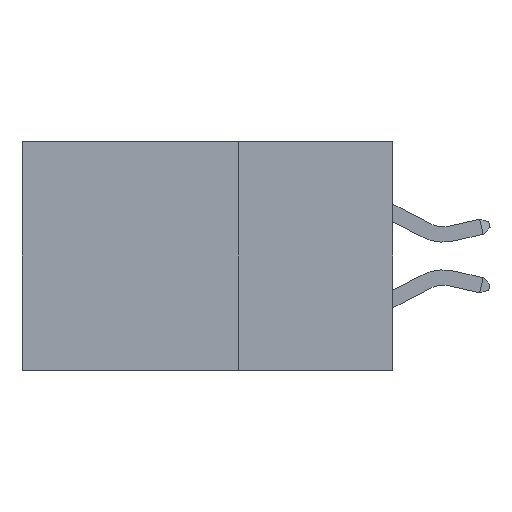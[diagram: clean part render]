
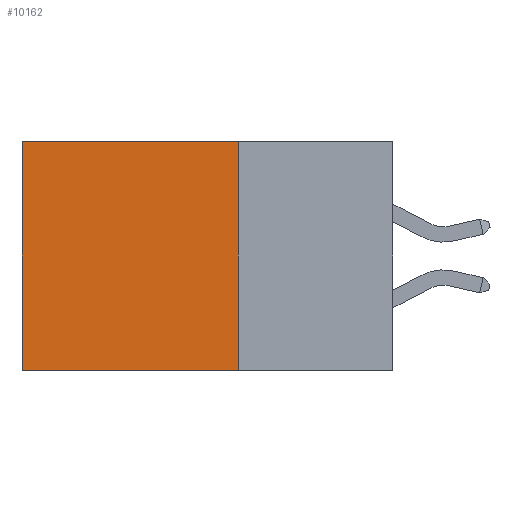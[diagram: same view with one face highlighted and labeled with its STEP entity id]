
A CAD part, left-side view. The second image highlights one B-rep face of the part: STEP entity #10162.
In plain terms, the highlighted planar face has unit normal (-1, 0, 0).
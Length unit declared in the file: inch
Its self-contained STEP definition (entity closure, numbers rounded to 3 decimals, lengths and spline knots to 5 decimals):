
#149 = DIRECTION ( 'NONE',  ( 0., 1., 0. ) ) ;
#296 = PLANE ( 'NONE',  #19587 ) ;
#452 = CARTESIAN_POINT ( 'NONE',  ( 0.2875, 0.6, 0. ) ) ;
#729 = FACE_OUTER_BOUND ( 'NONE', #6684, .T. ) ;
#1935 = EDGE_CURVE ( 'NONE', #9636, #14370, #9833, .T. ) ;
#1949 = VERTEX_POINT ( 'NONE', #7316 ) ;
#3012 = CARTESIAN_POINT ( 'NONE',  ( 0.2875, 0.25, 0. ) ) ;
#3735 = CARTESIAN_POINT ( 'NONE',  ( 0.2875, 0.25, 0. ) ) ;
#4680 = DIRECTION ( 'NONE',  ( 0., 1., 0. ) ) ;
#5199 = LINE ( 'NONE', #14654, #13036 ) ;
#6184 = VECTOR ( 'NONE', #7667, 39.37008 ) ;
#6657 = VECTOR ( 'NONE', #149, 39.37008 ) ;
#6684 = EDGE_LOOP ( 'NONE', ( #13046, #10165, #10647, #10287 ) ) ;
#7155 = DIRECTION ( 'NONE',  ( 0., 0., -1. ) ) ;
#7316 = CARTESIAN_POINT ( 'NONE',  ( 0.2875, 0.25, -0.37 ) ) ;
#7667 = DIRECTION ( 'NONE',  ( 0., 0., -1. ) ) ;
#8591 = CARTESIAN_POINT ( 'NONE',  ( 0.2875, 0.25, -0.37 ) ) ;
#9636 = VERTEX_POINT ( 'NONE', #17010 ) ;
#9833 = LINE ( 'NONE', #452, #14264 ) ;
#10162 = ADVANCED_FACE ( 'NONE', ( #729 ), #296, .F. ) ;
#10165 = ORIENTED_EDGE ( 'NONE', *, *, #20945, .F. ) ;
#10287 = ORIENTED_EDGE ( 'NONE', *, *, #15002, .T. ) ;
#10525 = LINE ( 'NONE', #8591, #6657 ) ;
#10605 = LINE ( 'NONE', #19178, #6184 ) ;
#10647 = ORIENTED_EDGE ( 'NONE', *, *, #16699, .F. ) ;
#12045 = VERTEX_POINT ( 'NONE', #3012 ) ;
#13036 = VECTOR ( 'NONE', #4680, 39.37008 ) ;
#13046 = ORIENTED_EDGE ( 'NONE', *, *, #1935, .T. ) ;
#14264 = VECTOR ( 'NONE', #18752, 39.37008 ) ;
#14370 = VERTEX_POINT ( 'NONE', #19574 ) ;
#14654 = CARTESIAN_POINT ( 'NONE',  ( 0.2875, 0.25, 0. ) ) ;
#15002 = EDGE_CURVE ( 'NONE', #12045, #9636, #5199, .T. ) ;
#16699 = EDGE_CURVE ( 'NONE', #12045, #1949, #10605, .T. ) ;
#17010 = CARTESIAN_POINT ( 'NONE',  ( 0.2875, 0.6, 0. ) ) ;
#17065 = DIRECTION ( 'NONE',  ( 1., 0., 0. ) ) ;
#18752 = DIRECTION ( 'NONE',  ( 0., 0., -1. ) ) ;
#19178 = CARTESIAN_POINT ( 'NONE',  ( 0.2875, 0.25, 0. ) ) ;
#19574 = CARTESIAN_POINT ( 'NONE',  ( 0.2875, 0.6, -0.37 ) ) ;
#19587 = AXIS2_PLACEMENT_3D ( 'NONE', #3735, #17065, #7155 ) ;
#20945 = EDGE_CURVE ( 'NONE', #1949, #14370, #10525, .T. ) ;
